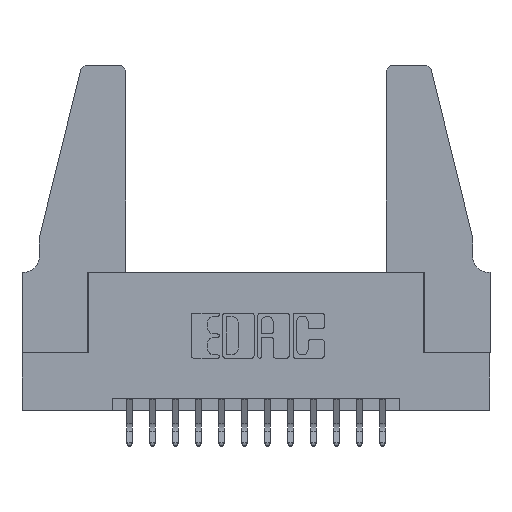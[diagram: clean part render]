
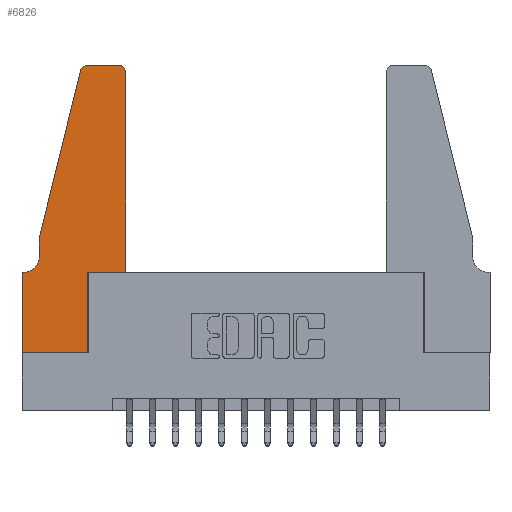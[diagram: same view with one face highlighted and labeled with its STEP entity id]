
A CAD part, top view. The second image highlights one B-rep face of the part: STEP entity #6826.
In plain terms, the highlighted planar face has unit normal (0, 0, 1).
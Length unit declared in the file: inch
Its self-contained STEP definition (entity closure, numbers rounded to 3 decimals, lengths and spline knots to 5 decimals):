
#92 = VERTEX_POINT ( 'NONE', #13201 ) ;
#138 = AXIS2_PLACEMENT_3D ( 'NONE', #2010, #9317, #3439 ) ;
#265 = DIRECTION ( 'NONE',  ( 1., 0., 0. ) ) ;
#273 = DIRECTION ( 'NONE',  ( 0., 1., 0. ) ) ;
#660 = CARTESIAN_POINT ( 'NONE',  ( 0.2605, 1.25, 0.37 ) ) ;
#875 = ORIENTED_EDGE ( 'NONE', *, *, #10499, .T. ) ;
#895 = VERTEX_POINT ( 'NONE', #12125 ) ;
#902 = VECTOR ( 'NONE', #6819, 39.37008 ) ;
#1189 = VECTOR ( 'NONE', #3703, 39.37008 ) ;
#1191 = EDGE_CURVE ( 'NONE', #5906, #2471, #15402, .T. ) ;
#1793 = AXIS2_PLACEMENT_3D ( 'NONE', #2068, #3400, #12049 ) ;
#1921 = DIRECTION ( 'NONE',  ( -1., 0., 0. ) ) ;
#2010 = CARTESIAN_POINT ( 'NONE',  ( 0.284, 1.22, 0.37 ) ) ;
#2068 = CARTESIAN_POINT ( 'NONE',  ( 0., 0.35, 0.37 ) ) ;
#2129 = LINE ( 'NONE', #14989, #11690 ) ;
#2278 = CIRCLE ( 'NONE', #4038, 0.07 ) ;
#2471 = VERTEX_POINT ( 'NONE', #14510 ) ;
#2518 = AXIS2_PLACEMENT_3D ( 'NONE', #14979, #7929, #265 ) ;
#2552 = VECTOR ( 'NONE', #7733, 39.37008 ) ;
#2612 = CARTESIAN_POINT ( 'NONE',  ( 0., 0., 0.37 ) ) ;
#2886 = CARTESIAN_POINT ( 'NONE',  ( 0.2865, 0.35, 0.37 ) ) ;
#3157 = VERTEX_POINT ( 'NONE', #12279 ) ;
#3226 = VECTOR ( 'NONE', #14830, 39.37008 ) ;
#3240 = CARTESIAN_POINT ( 'NONE',  ( 0.0755, 0.42, 0.37 ) ) ;
#3400 = DIRECTION ( 'NONE',  ( 0., 0., 1. ) ) ;
#3439 = DIRECTION ( 'NONE',  ( 1., 0., 0. ) ) ;
#3455 = VERTEX_POINT ( 'NONE', #2886 ) ;
#3499 = ORIENTED_EDGE ( 'NONE', *, *, #8019, .T. ) ;
#3703 = DIRECTION ( 'NONE',  ( 0., 1., 0. ) ) ;
#3711 = CARTESIAN_POINT ( 'NONE',  ( 0.0755, 0.35, 0.37 ) ) ;
#4038 = AXIS2_PLACEMENT_3D ( 'NONE', #4509, #13011, #5781 ) ;
#4296 = EDGE_CURVE ( 'NONE', #2471, #895, #13490, .T. ) ;
#4509 = CARTESIAN_POINT ( 'NONE',  ( 0.0055, 0.42, 0.37 ) ) ;
#4736 = ORIENTED_EDGE ( 'NONE', *, *, #5642, .T. ) ;
#4953 = VECTOR ( 'NONE', #11161, 39.37008 ) ;
#5118 = ORIENTED_EDGE ( 'NONE', *, *, #13538, .T. ) ;
#5555 = CARTESIAN_POINT ( 'NONE',  ( 0.0755, 0.5, 0.37 ) ) ;
#5642 = EDGE_CURVE ( 'NONE', #12250, #6987, #8292, .T. ) ;
#5781 = DIRECTION ( 'NONE',  ( -1., 0., 0. ) ) ;
#5906 = VERTEX_POINT ( 'NONE', #7981 ) ;
#5923 = ORIENTED_EDGE ( 'NONE', *, *, #8253, .T. ) ;
#6506 = CARTESIAN_POINT ( 'NONE',  ( 0., 0., 0.37 ) ) ;
#6819 = DIRECTION ( 'NONE',  ( 0., -1., 0. ) ) ;
#6826 = ADVANCED_FACE ( 'NONE', ( #14315 ), #9699, .T. ) ;
#6987 = VERTEX_POINT ( 'NONE', #7531 ) ;
#7033 = CARTESIAN_POINT ( 'NONE',  ( 0.0755, 0.5, 0.37 ) ) ;
#7101 = VERTEX_POINT ( 'NONE', #14795 ) ;
#7292 = ORIENTED_EDGE ( 'NONE', *, *, #4296, .T. ) ;
#7531 = CARTESIAN_POINT ( 'NONE',  ( 0., 0.35, 0.37 ) ) ;
#7679 = ORIENTED_EDGE ( 'NONE', *, *, #10605, .T. ) ;
#7733 = DIRECTION ( 'NONE',  ( 0., -1., 0. ) ) ;
#7929 = DIRECTION ( 'NONE',  ( 0., 0., 1. ) ) ;
#7981 = CARTESIAN_POINT ( 'NONE',  ( 0.284, 1.25, 0.37 ) ) ;
#8019 = EDGE_CURVE ( 'NONE', #92, #5906, #11754, .T. ) ;
#8060 = VECTOR ( 'NONE', #14023, 39.37008 ) ;
#8253 = EDGE_CURVE ( 'NONE', #3157, #7101, #14275, .T. ) ;
#8292 = LINE ( 'NONE', #3711, #4953 ) ;
#8475 = ORIENTED_EDGE ( 'NONE', *, *, #9817, .T. ) ;
#8842 = ORIENTED_EDGE ( 'NONE', *, *, #11326, .T. ) ;
#9317 = DIRECTION ( 'NONE',  ( 0., 0., 1. ) ) ;
#9532 = DIRECTION ( 'NONE',  ( -0.239, -0.971, 0. ) ) ;
#9699 = PLANE ( 'NONE',  #1793 ) ;
#9817 = EDGE_CURVE ( 'NONE', #12580, #3455, #2129, .T. ) ;
#9919 = CARTESIAN_POINT ( 'NONE',  ( 0.0055, 0.35, 0.37 ) ) ;
#9975 = CARTESIAN_POINT ( 'NONE',  ( 0.4505, 0.35, 0.37 ) ) ;
#10070 = CARTESIAN_POINT ( 'NONE',  ( 0., 0., 0.37 ) ) ;
#10499 = EDGE_CURVE ( 'NONE', #895, #12050, #13627, .T. ) ;
#10605 = EDGE_CURVE ( 'NONE', #12050, #12250, #2278, .T. ) ;
#10721 = CARTESIAN_POINT ( 'NONE',  ( 0.2865, 0., 0.37 ) ) ;
#10777 = VECTOR ( 'NONE', #9532, 39.37008 ) ;
#11161 = DIRECTION ( 'NONE',  ( -1., 0., 0. ) ) ;
#11271 = ORIENTED_EDGE ( 'NONE', *, *, #14656, .T. ) ;
#11326 = EDGE_CURVE ( 'NONE', #3455, #3157, #14335, .T. ) ;
#11690 = VECTOR ( 'NONE', #273, 39.37008 ) ;
#11754 = LINE ( 'NONE', #660, #14087 ) ;
#11939 = CIRCLE ( 'NONE', #2518, 0.03 ) ;
#12049 = DIRECTION ( 'NONE',  ( 1., 0., 0. ) ) ;
#12050 = VERTEX_POINT ( 'NONE', #3240 ) ;
#12125 = CARTESIAN_POINT ( 'NONE',  ( 0.0755, 0.5, 0.37 ) ) ;
#12250 = VERTEX_POINT ( 'NONE', #9919 ) ;
#12279 = CARTESIAN_POINT ( 'NONE',  ( 0.4505, 0.35, 0.37 ) ) ;
#12364 = ORIENTED_EDGE ( 'NONE', *, *, #13608, .T. ) ;
#12580 = VERTEX_POINT ( 'NONE', #10721 ) ;
#12886 = CARTESIAN_POINT ( 'NONE',  ( 0.4505, 0.35, 0.37 ) ) ;
#13011 = DIRECTION ( 'NONE',  ( 0., 0., -1. ) ) ;
#13201 = CARTESIAN_POINT ( 'NONE',  ( 0.4205, 1.25, 0.37 ) ) ;
#13260 = ORIENTED_EDGE ( 'NONE', *, *, #1191, .T. ) ;
#13490 = LINE ( 'NONE', #7033, #10777 ) ;
#13538 = EDGE_CURVE ( 'NONE', #15200, #12580, #15715, .T. ) ;
#13608 = EDGE_CURVE ( 'NONE', #7101, #92, #11939, .T. ) ;
#13627 = LINE ( 'NONE', #5555, #902 ) ;
#14023 = DIRECTION ( 'NONE',  ( 1., 0., 0. ) ) ;
#14087 = VECTOR ( 'NONE', #1921, 39.37008 ) ;
#14275 = LINE ( 'NONE', #9975, #1189 ) ;
#14315 = FACE_OUTER_BOUND ( 'NONE', #15536, .T. ) ;
#14335 = LINE ( 'NONE', #12886, #8060 ) ;
#14510 = CARTESIAN_POINT ( 'NONE',  ( 0.25487, 1.22718, 0.37 ) ) ;
#14656 = EDGE_CURVE ( 'NONE', #6987, #15200, #15855, .T. ) ;
#14795 = CARTESIAN_POINT ( 'NONE',  ( 0.4505, 1.22, 0.37 ) ) ;
#14830 = DIRECTION ( 'NONE',  ( 1., 0., 0. ) ) ;
#14979 = CARTESIAN_POINT ( 'NONE',  ( 0.4205, 1.22, 0.37 ) ) ;
#14989 = CARTESIAN_POINT ( 'NONE',  ( 0.2865, 0.35, 0.37 ) ) ;
#15200 = VERTEX_POINT ( 'NONE', #10070 ) ;
#15402 = CIRCLE ( 'NONE', #138, 0.03 ) ;
#15536 = EDGE_LOOP ( 'NONE', ( #3499, #13260, #7292, #875, #7679, #4736, #11271, #5118, #8475, #8842, #5923, #12364 ) ) ;
#15715 = LINE ( 'NONE', #6506, #3226 ) ;
#15855 = LINE ( 'NONE', #2612, #2552 ) ;
